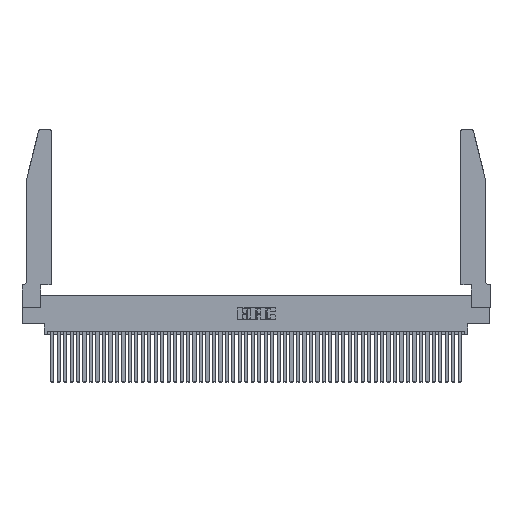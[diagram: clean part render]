
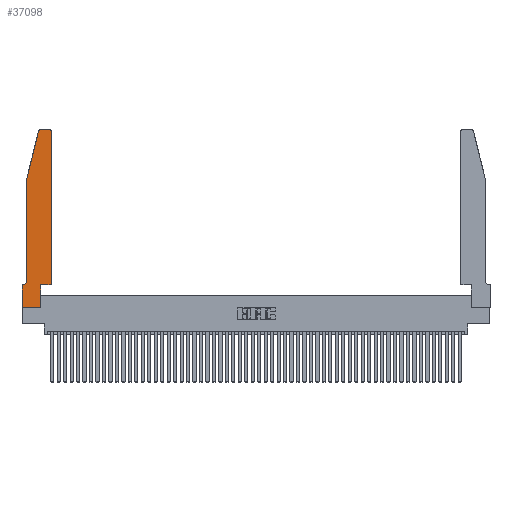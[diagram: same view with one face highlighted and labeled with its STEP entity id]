
A CAD part, top view. The second image highlights one B-rep face of the part: STEP entity #37098.
In plain terms, the highlighted planar face has unit normal (0, 0, 1).
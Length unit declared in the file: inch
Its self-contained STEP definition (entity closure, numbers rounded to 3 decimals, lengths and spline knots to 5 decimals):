
#63 = EDGE_CURVE ( 'NONE', #4610, #1171, #20722, .T. ) ;
#143 = EDGE_CURVE ( 'NONE', #46043, #32427, #48895, .T. ) ;
#852 = CARTESIAN_POINT ( 'NONE',  ( 0.0755, 2., 0.37 ) ) ;
#1005 = EDGE_CURVE ( 'NONE', #17456, #49321, #23151, .T. ) ;
#1171 = VERTEX_POINT ( 'NONE', #47999 ) ;
#2695 = LINE ( 'NONE', #32568, #22828 ) ;
#3031 = EDGE_CURVE ( 'NONE', #27275, #14149, #16553, .T. ) ;
#3059 = CARTESIAN_POINT ( 'NONE',  ( 0., 0.35, 0.37 ) ) ;
#3275 = EDGE_CURVE ( 'NONE', #14149, #4610, #26611, .T. ) ;
#4403 = VERTEX_POINT ( 'NONE', #21351 ) ;
#4610 = VERTEX_POINT ( 'NONE', #6367 ) ;
#4835 = VECTOR ( 'NONE', #20939, 39.37008 ) ;
#5098 = CARTESIAN_POINT ( 'NONE',  ( 0., 0., 0.37 ) ) ;
#6367 = CARTESIAN_POINT ( 'NONE',  ( 0.284, 2.75, 0.37 ) ) ;
#6517 = LINE ( 'NONE', #21330, #25425 ) ;
#6723 = VERTEX_POINT ( 'NONE', #7976 ) ;
#6760 = DIRECTION ( 'NONE',  ( 0., 0., 1. ) ) ;
#7003 = CARTESIAN_POINT ( 'NONE',  ( 0.4205, 2.72, 0.37 ) ) ;
#7342 = LINE ( 'NONE', #852, #4835 ) ;
#7976 = CARTESIAN_POINT ( 'NONE',  ( 0.2865, 0., 0.37 ) ) ;
#8869 = ORIENTED_EDGE ( 'NONE', *, *, #143, .T. ) ;
#9198 = CARTESIAN_POINT ( 'NONE',  ( 0.284, 2.72, 0.37 ) ) ;
#10014 = AXIS2_PLACEMENT_3D ( 'NONE', #46560, #6760, #34834 ) ;
#10288 = AXIS2_PLACEMENT_3D ( 'NONE', #19515, #47523, #23582 ) ;
#10650 = EDGE_CURVE ( 'NONE', #4403, #27275, #32175, .T. ) ;
#10830 = VECTOR ( 'NONE', #24369, 39.37008 ) ;
#11042 = DIRECTION ( 'NONE',  ( 1., 0., 0. ) ) ;
#12786 = ORIENTED_EDGE ( 'NONE', *, *, #3275, .T. ) ;
#13223 = DIRECTION ( 'NONE',  ( 1., 0., 0. ) ) ;
#14149 = VERTEX_POINT ( 'NONE', #16135 ) ;
#16069 = CARTESIAN_POINT ( 'NONE',  ( 0.4505, 2.72, 0.37 ) ) ;
#16135 = CARTESIAN_POINT ( 'NONE',  ( 0.4205, 2.75, 0.37 ) ) ;
#16484 = DIRECTION ( 'NONE',  ( -1., 0., 0. ) ) ;
#16553 = CIRCLE ( 'NONE', #45563, 0.03 ) ;
#16595 = DIRECTION ( 'NONE',  ( 1., 0., 0. ) ) ;
#17456 = VERTEX_POINT ( 'NONE', #41861 ) ;
#19388 = CARTESIAN_POINT ( 'NONE',  ( 0.2865, 0.35, 0.37 ) ) ;
#19418 = EDGE_CURVE ( 'NONE', #35720, #6723, #2695, .T. ) ;
#19515 = CARTESIAN_POINT ( 'NONE',  ( 0.0055, 0.42, 0.37 ) ) ;
#19985 = ORIENTED_EDGE ( 'NONE', *, *, #23064, .T. ) ;
#20153 = LINE ( 'NONE', #5098, #37698 ) ;
#20286 = CARTESIAN_POINT ( 'NONE',  ( 0.4505, 0.35, 0.37 ) ) ;
#20722 = CIRCLE ( 'NONE', #50169, 0.03 ) ;
#20939 = DIRECTION ( 'NONE',  ( -0.239, -0.971, 0. ) ) ;
#21330 = CARTESIAN_POINT ( 'NONE',  ( 0.4505, 0.35, 0.37 ) ) ;
#21351 = CARTESIAN_POINT ( 'NONE',  ( 0.4505, 0.35, 0.37 ) ) ;
#22828 = VECTOR ( 'NONE', #16595, 39.37008 ) ;
#22953 = ORIENTED_EDGE ( 'NONE', *, *, #32268, .T. ) ;
#23064 = EDGE_CURVE ( 'NONE', #6723, #38563, #45278, .T. ) ;
#23151 = LINE ( 'NONE', #39075, #41889 ) ;
#23582 = DIRECTION ( 'NONE',  ( -1., 0., 0. ) ) ;
#24369 = DIRECTION ( 'NONE',  ( 0., 1., 0. ) ) ;
#25273 = ORIENTED_EDGE ( 'NONE', *, *, #1005, .T. ) ;
#25425 = VECTOR ( 'NONE', #37233, 39.37008 ) ;
#25488 = ORIENTED_EDGE ( 'NONE', *, *, #48249, .T. ) ;
#26611 = LINE ( 'NONE', #28633, #47836 ) ;
#27240 = ORIENTED_EDGE ( 'NONE', *, *, #35158, .T. ) ;
#27275 = VERTEX_POINT ( 'NONE', #16069 ) ;
#27426 = ORIENTED_EDGE ( 'NONE', *, *, #10650, .T. ) ;
#27623 = ORIENTED_EDGE ( 'NONE', *, *, #3031, .T. ) ;
#27648 = VECTOR ( 'NONE', #49698, 39.37008 ) ;
#28633 = CARTESIAN_POINT ( 'NONE',  ( 0.2605, 2.75, 0.37 ) ) ;
#29345 = DIRECTION ( 'NONE',  ( 0., -1., 0. ) ) ;
#30212 = EDGE_LOOP ( 'NONE', ( #12786, #37457, #27240, #8869, #25488, #25273, #22953, #30769, #19985, #32662, #27426, #27623 ) ) ;
#30305 = EDGE_CURVE ( 'NONE', #38563, #4403, #6517, .T. ) ;
#30769 = ORIENTED_EDGE ( 'NONE', *, *, #19418, .T. ) ;
#31327 = DIRECTION ( 'NONE',  ( 0., 1., 0. ) ) ;
#32175 = LINE ( 'NONE', #20286, #10830 ) ;
#32268 = EDGE_CURVE ( 'NONE', #49321, #35720, #20153, .T. ) ;
#32346 = FACE_OUTER_BOUND ( 'NONE', #30212, .T. ) ;
#32427 = VERTEX_POINT ( 'NONE', #34214 ) ;
#32568 = CARTESIAN_POINT ( 'NONE',  ( 0., 0., 0.37 ) ) ;
#32662 = ORIENTED_EDGE ( 'NONE', *, *, #30305, .T. ) ;
#33072 = CARTESIAN_POINT ( 'NONE',  ( 0.0755, 2., 0.37 ) ) ;
#34214 = CARTESIAN_POINT ( 'NONE',  ( 0.0755, 0.42, 0.37 ) ) ;
#34646 = VECTOR ( 'NONE', #31327, 39.37008 ) ;
#34834 = DIRECTION ( 'NONE',  ( 1., 0., 0. ) ) ;
#35081 = DIRECTION ( 'NONE',  ( 0., 0., 1. ) ) ;
#35158 = EDGE_CURVE ( 'NONE', #1171, #46043, #7342, .T. ) ;
#35720 = VERTEX_POINT ( 'NONE', #40630 ) ;
#37098 = ADVANCED_FACE ( 'NONE', ( #32346 ), #50774, .T. ) ;
#37233 = DIRECTION ( 'NONE',  ( 1., 0., 0. ) ) ;
#37260 = DIRECTION ( 'NONE',  ( 0., 0., 1. ) ) ;
#37457 = ORIENTED_EDGE ( 'NONE', *, *, #63, .T. ) ;
#37698 = VECTOR ( 'NONE', #29345, 39.37008 ) ;
#38563 = VERTEX_POINT ( 'NONE', #39580 ) ;
#39075 = CARTESIAN_POINT ( 'NONE',  ( 0.0755, 0.35, 0.37 ) ) ;
#39580 = CARTESIAN_POINT ( 'NONE',  ( 0.2865, 0.35, 0.37 ) ) ;
#40630 = CARTESIAN_POINT ( 'NONE',  ( 0., 0., 0.37 ) ) ;
#41861 = CARTESIAN_POINT ( 'NONE',  ( 0.0055, 0.35, 0.37 ) ) ;
#41889 = VECTOR ( 'NONE', #43113, 39.37008 ) ;
#43113 = DIRECTION ( 'NONE',  ( -1., 0., 0. ) ) ;
#45278 = LINE ( 'NONE', #19388, #34646 ) ;
#45563 = AXIS2_PLACEMENT_3D ( 'NONE', #7003, #35081, #11042 ) ;
#45657 = CARTESIAN_POINT ( 'NONE',  ( 0.0755, 2., 0.37 ) ) ;
#46043 = VERTEX_POINT ( 'NONE', #33072 ) ;
#46560 = CARTESIAN_POINT ( 'NONE',  ( 0., 0.35, 0.37 ) ) ;
#47523 = DIRECTION ( 'NONE',  ( 0., 0., -1. ) ) ;
#47643 = CIRCLE ( 'NONE', #10288, 0.07 ) ;
#47836 = VECTOR ( 'NONE', #16484, 39.37008 ) ;
#47999 = CARTESIAN_POINT ( 'NONE',  ( 0.25487, 2.72718, 0.37 ) ) ;
#48249 = EDGE_CURVE ( 'NONE', #32427, #17456, #47643, .T. ) ;
#48895 = LINE ( 'NONE', #45657, #27648 ) ;
#49321 = VERTEX_POINT ( 'NONE', #3059 ) ;
#49698 = DIRECTION ( 'NONE',  ( 0., -1., 0. ) ) ;
#50169 = AXIS2_PLACEMENT_3D ( 'NONE', #9198, #37260, #13223 ) ;
#50774 = PLANE ( 'NONE',  #10014 ) ;
